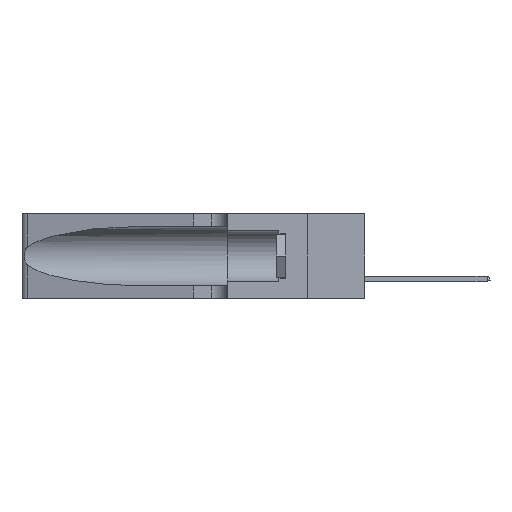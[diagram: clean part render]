
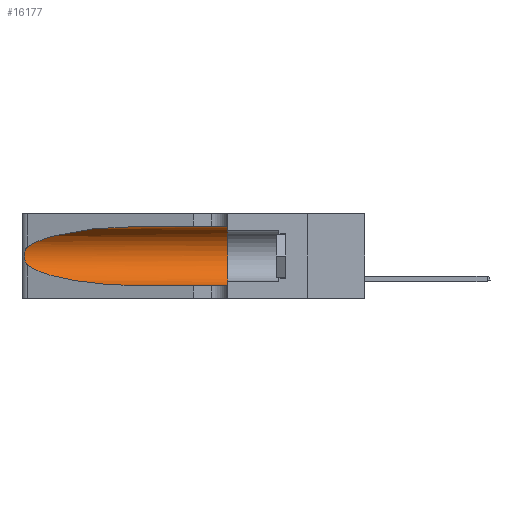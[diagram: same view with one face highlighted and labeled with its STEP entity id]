
A CAD part, left-side view. The second image highlights one B-rep face of the part: STEP entity #16177.
In plain terms, the highlighted cylindrical face has radius 3.308 mm (diameter 6.617 mm), a partial arc.
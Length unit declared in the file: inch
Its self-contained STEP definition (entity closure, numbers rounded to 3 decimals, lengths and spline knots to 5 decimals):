
#274 = CARTESIAN_POINT ( 'NONE',  ( 0.25487, 1.22718, 0.22369 ) ) ;
#299 = CARTESIAN_POINT ( 'NONE',  ( 0.26075, 1.23896, 0.178 ) ) ;
#323 = CARTESIAN_POINT ( 'NONE',  ( 0.18966, 0.96281, 0.05475 ) ) ;
#648 = CIRCLE ( 'NONE', #6277, 0.13025 ) ;
#661 = ORIENTED_EDGE ( 'NONE', *, *, #5271, .F. ) ;
#663 = EDGE_CURVE ( 'NONE', #13667, #7452, #20597, .T. ) ;
#1039 = CARTESIAN_POINT ( 'NONE',  ( 0.1305, 0.72297, 0.05475 ) ) ;
#1336 = VECTOR ( 'NONE', #7831, 39.37008 ) ;
#3130 = CARTESIAN_POINT ( 'NONE',  ( 0.25639, 1.23184, 0.21858 ) ) ;
#3637 = CARTESIAN_POINT ( 'NONE',  ( 0.25487, 1.22718, 0.14631 ) ) ;
#3979 = AXIS2_PLACEMENT_3D ( 'NONE', #13542, #17058, #11864 ) ;
#4026 = CARTESIAN_POINT ( 'NONE',  ( 0.25555, 1.22993, 0.14849 ) ) ;
#5095 = CARTESIAN_POINT ( 'NONE',  ( 0.26075, 1.23896, 0.19203 ) ) ;
#5271 = EDGE_CURVE ( 'NONE', #9655, #10592, #10640, .T. ) ;
#5360 = CARTESIAN_POINT ( 'NONE',  ( 0.18966, 0.96281, 0.31525 ) ) ;
#5658 = EDGE_CURVE ( 'NONE', #7452, #15245, #20990, .T. ) ;
#5693 = DIRECTION ( 'NONE',  ( 0., 1., 0. ) ) ;
#5734 = CARTESIAN_POINT ( 'NONE',  ( 0.26017, 1.23833, 0.17102 ) ) ;
#5875 = DIRECTION ( 'NONE',  ( 0., -1., 0. ) ) ;
#6277 = AXIS2_PLACEMENT_3D ( 'NONE', #10876, #5693, #19706 ) ;
#7281 =( BOUNDED_CURVE ( )  B_SPLINE_CURVE ( 3, ( #10767, #5360, #21378, #274 ),
 .UNSPECIFIED., .F., .F. ) 
 B_SPLINE_CURVE_WITH_KNOTS ( ( 4, 4 ),
 ( 1.5708, 2.84003 ),
 .UNSPECIFIED. ) 
 CURVE ( )  GEOMETRIC_REPRESENTATION_ITEM ( )  RATIONAL_B_SPLINE_CURVE ( ( 1., 0.87, 0.87, 1. ) ) 
 REPRESENTATION_ITEM ( '' )  );
#7345 = FACE_OUTER_BOUND ( 'NONE', #15448, .T. ) ;
#7353 = CARTESIAN_POINT ( 'NONE',  ( 0.25487, 1.22718, 0.14631 ) ) ;
#7445 = CARTESIAN_POINT ( 'NONE',  ( 0.25487, 1.22718, 0.14631 ) ) ;
#7452 = VERTEX_POINT ( 'NONE', #1039 ) ;
#7628 = CARTESIAN_POINT ( 'NONE',  ( 0.1305, 1.61858, 0.05475 ) ) ;
#7831 = DIRECTION ( 'NONE',  ( 0., -1., 0. ) ) ;
#8331 = CARTESIAN_POINT ( 'NONE',  ( 0.25487, 1.22718, 0.22369 ) ) ;
#8333 = ORIENTED_EDGE ( 'NONE', *, *, #14238, .T. ) ;
#8575 = ORIENTED_EDGE ( 'NONE', *, *, #22620, .T. ) ;
#8666 = VERTEX_POINT ( 'NONE', #20347 ) ;
#9606 = ORIENTED_EDGE ( 'NONE', *, *, #12195, .F. ) ;
#9655 = VERTEX_POINT ( 'NONE', #21417 ) ;
#10592 = VERTEX_POINT ( 'NONE', #13755 ) ;
#10640 = LINE ( 'NONE', #21570, #1336 ) ;
#10767 = CARTESIAN_POINT ( 'NONE',  ( 0.1305, 0.72297, 0.31525 ) ) ;
#10876 = CARTESIAN_POINT ( 'NONE',  ( 0.1305, 0.35, 0.185 ) ) ;
#10926 = CARTESIAN_POINT ( 'NONE',  ( 0.25639, 1.23186, 0.15144 ) ) ;
#11864 = DIRECTION ( 'NONE',  ( 0., 0., -1. ) ) ;
#12195 = EDGE_CURVE ( 'NONE', #10592, #15245, #648, .T. ) ;
#12356 = CARTESIAN_POINT ( 'NONE',  ( 0.26018, 1.23835, 0.19895 ) ) ;
#12537 = CARTESIAN_POINT ( 'NONE',  ( 0.25789, 1.23486, 0.15765 ) ) ;
#13542 = CARTESIAN_POINT ( 'NONE',  ( 0.1305, 1.61858, 0.185 ) ) ;
#13599 = CARTESIAN_POINT ( 'NONE',  ( 0.25555, 1.22994, 0.2215 ) ) ;
#13613 = CARTESIAN_POINT ( 'NONE',  ( 0.1305, 0.35, 0.05475 ) ) ;
#13667 = VERTEX_POINT ( 'NONE', #7445 ) ;
#13755 = CARTESIAN_POINT ( 'NONE',  ( 0.1305, 0.35, 0.31525 ) ) ;
#13882 = VECTOR ( 'NONE', #5875, 39.37008 ) ;
#14238 = EDGE_CURVE ( 'NONE', #8666, #13667, #14536, .T. ) ;
#14536 = B_SPLINE_CURVE_WITH_KNOTS ( 'NONE', 3,
 ( #8331, #13599, #3130, #15327, #17560, #12356, #5095, #299, #5734, #17741, #12537, #10926, #4026, #7353 ),
 .UNSPECIFIED., .F., .F.,
 ( 4, 2, 2, 2, 2, 2, 4 ),
 ( 0., 0.00027, 0.00053, 0.00107, 0.0016, 0.00187, 0.00214 ),
 .UNSPECIFIED. ) ;
#15245 = VERTEX_POINT ( 'NONE', #13613 ) ;
#15327 = CARTESIAN_POINT ( 'NONE',  ( 0.25787, 1.23484, 0.2124 ) ) ;
#15448 = EDGE_LOOP ( 'NONE', ( #8575, #8333, #17798, #21303, #9606, #661 ) ) ;
#15846 = CARTESIAN_POINT ( 'NONE',  ( 0.2373, 1.15595, 0.08982 ) ) ;
#16177 = ADVANCED_FACE ( 'NONE', ( #7345 ), #18278, .F. ) ;
#17058 = DIRECTION ( 'NONE',  ( 0., -1., 0. ) ) ;
#17560 = CARTESIAN_POINT ( 'NONE',  ( 0.25854, 1.2359, 0.20912 ) ) ;
#17741 = CARTESIAN_POINT ( 'NONE',  ( 0.25856, 1.23593, 0.16098 ) ) ;
#17798 = ORIENTED_EDGE ( 'NONE', *, *, #663, .T. ) ;
#18278 = CYLINDRICAL_SURFACE ( 'NONE', #3979, 0.13025 ) ;
#19706 = DIRECTION ( 'NONE',  ( 0., 0., 1. ) ) ;
#20347 = CARTESIAN_POINT ( 'NONE',  ( 0.25487, 1.22718, 0.22369 ) ) ;
#20597 =( BOUNDED_CURVE ( )  B_SPLINE_CURVE ( 3, ( #3637, #15846, #323, #20998 ),
 .UNSPECIFIED., .F., .F. ) 
 B_SPLINE_CURVE_WITH_KNOTS ( ( 4, 4 ),
 ( 3.44316, 4.71239 ),
 .UNSPECIFIED. ) 
 CURVE ( )  GEOMETRIC_REPRESENTATION_ITEM ( )  RATIONAL_B_SPLINE_CURVE ( ( 1., 0.87, 0.87, 1. ) ) 
 REPRESENTATION_ITEM ( '' )  );
#20990 = LINE ( 'NONE', #7628, #13882 ) ;
#20998 = CARTESIAN_POINT ( 'NONE',  ( 0.1305, 0.72297, 0.05475 ) ) ;
#21303 = ORIENTED_EDGE ( 'NONE', *, *, #5658, .T. ) ;
#21378 = CARTESIAN_POINT ( 'NONE',  ( 0.2373, 1.15595, 0.28018 ) ) ;
#21417 = CARTESIAN_POINT ( 'NONE',  ( 0.1305, 0.72297, 0.31525 ) ) ;
#21570 = CARTESIAN_POINT ( 'NONE',  ( 0.1305, 1.61858, 0.31525 ) ) ;
#22620 = EDGE_CURVE ( 'NONE', #9655, #8666, #7281, .T. ) ;
